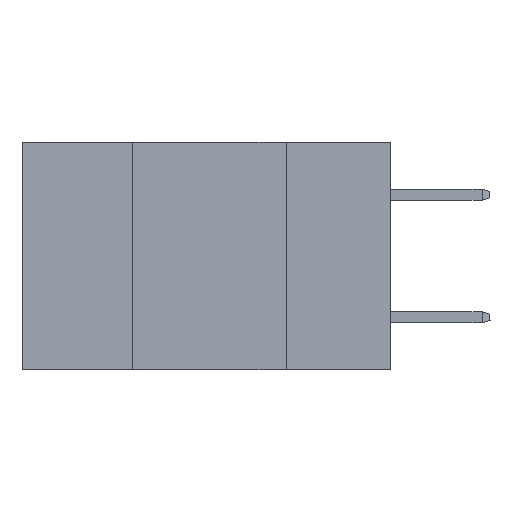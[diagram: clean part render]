
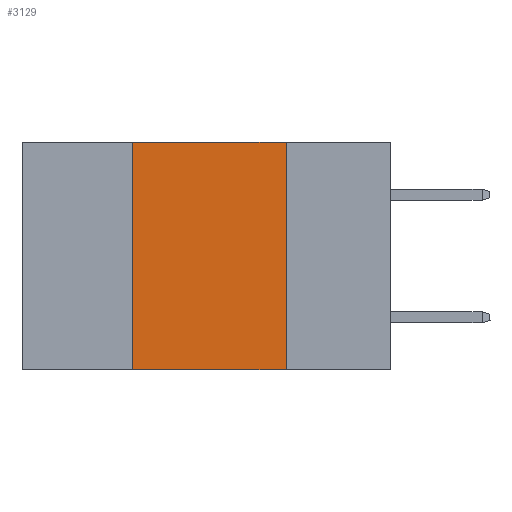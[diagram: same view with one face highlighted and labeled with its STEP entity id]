
A CAD part, left-side view. The second image highlights one B-rep face of the part: STEP entity #3129.
In plain terms, the highlighted planar face has unit normal (-1, 0, 0).
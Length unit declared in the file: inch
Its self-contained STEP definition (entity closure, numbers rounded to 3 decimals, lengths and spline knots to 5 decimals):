
#21 = ORIENTED_EDGE ( 'NONE', *, *, #3226, .F. ) ;
#665 = VERTEX_POINT ( 'NONE', #17845 ) ;
#1096 = VERTEX_POINT ( 'NONE', #24529 ) ;
#1965 = FACE_OUTER_BOUND ( 'NONE', #8662, .T. ) ;
#2484 = ORIENTED_EDGE ( 'NONE', *, *, #20855, .F. ) ;
#2695 = LINE ( 'NONE', #10903, #26253 ) ;
#3129 = ADVANCED_FACE ( 'NONE', ( #1965 ), #9168, .F. ) ;
#3226 = EDGE_CURVE ( 'NONE', #1096, #665, #17512, .T. ) ;
#4579 = LINE ( 'NONE', #15109, #10508 ) ;
#4767 = DIRECTION ( 'NONE',  ( 0., 0., -1. ) ) ;
#4897 = AXIS2_PLACEMENT_3D ( 'NONE', #26774, #18011, #4767 ) ;
#7077 = ORIENTED_EDGE ( 'NONE', *, *, #16371, .F. ) ;
#8662 = EDGE_LOOP ( 'NONE', ( #2484, #21, #7077, #17720 ) ) ;
#9168 = PLANE ( 'NONE',  #4897 ) ;
#10508 = VECTOR ( 'NONE', #28289, 39.37008 ) ;
#10903 = CARTESIAN_POINT ( 'NONE',  ( 0., 0.17, 0. ) ) ;
#11547 = DIRECTION ( 'NONE',  ( 0., -1., 0. ) ) ;
#11658 = DIRECTION ( 'NONE',  ( 0., -1., 0. ) ) ;
#11683 = VECTOR ( 'NONE', #11658, 39.37008 ) ;
#13608 = CARTESIAN_POINT ( 'NONE',  ( 0., 0.42, -0.37 ) ) ;
#13738 = CARTESIAN_POINT ( 'NONE',  ( 0., 0.17, -0.37 ) ) ;
#15109 = CARTESIAN_POINT ( 'NONE',  ( 0., 0.42, 0. ) ) ;
#16371 = EDGE_CURVE ( 'NONE', #27146, #1096, #4579, .T. ) ;
#17512 = LINE ( 'NONE', #24876, #11683 ) ;
#17720 = ORIENTED_EDGE ( 'NONE', *, *, #19929, .T. ) ;
#17845 = CARTESIAN_POINT ( 'NONE',  ( 0., 0.17, 0. ) ) ;
#18011 = DIRECTION ( 'NONE',  ( 1., 0., 0. ) ) ;
#19929 = EDGE_CURVE ( 'NONE', #27146, #24135, #21481, .T. ) ;
#20855 = EDGE_CURVE ( 'NONE', #665, #24135, #2695, .T. ) ;
#21481 = LINE ( 'NONE', #24758, #26593 ) ;
#24135 = VERTEX_POINT ( 'NONE', #13738 ) ;
#24529 = CARTESIAN_POINT ( 'NONE',  ( 0., 0.42, 0. ) ) ;
#24758 = CARTESIAN_POINT ( 'NONE',  ( 0., 0.6, -0.37 ) ) ;
#24876 = CARTESIAN_POINT ( 'NONE',  ( 0., 0.6, 0. ) ) ;
#26253 = VECTOR ( 'NONE', #26309, 39.37008 ) ;
#26309 = DIRECTION ( 'NONE',  ( 0., 0., -1. ) ) ;
#26593 = VECTOR ( 'NONE', #11547, 39.37008 ) ;
#26774 = CARTESIAN_POINT ( 'NONE',  ( 0., 0.6, 0. ) ) ;
#27146 = VERTEX_POINT ( 'NONE', #13608 ) ;
#28289 = DIRECTION ( 'NONE',  ( 0., 0., 1. ) ) ;
